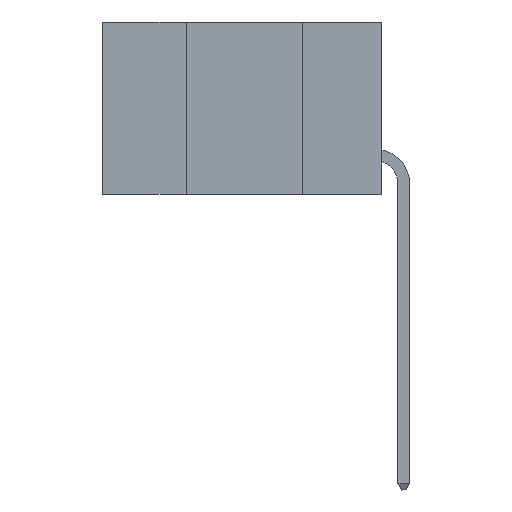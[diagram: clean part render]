
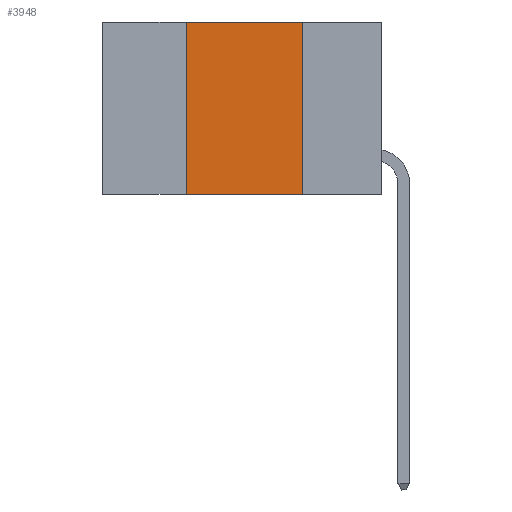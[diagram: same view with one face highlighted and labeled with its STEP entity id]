
A CAD part, left-side view. The second image highlights one B-rep face of the part: STEP entity #3948.
In plain terms, the highlighted planar face has unit normal (-1, 0, 0).
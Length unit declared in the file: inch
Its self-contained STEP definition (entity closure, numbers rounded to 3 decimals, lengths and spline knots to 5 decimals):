
#1010 = LINE ( 'NONE', #6924, #2339 ) ;
#1045 = DIRECTION ( 'NONE',  ( 1., 0., 0. ) ) ;
#1065 = ORIENTED_EDGE ( 'NONE', *, *, #8883, .F. ) ;
#1316 = CARTESIAN_POINT ( 'NONE',  ( 0., 0.17, 0. ) ) ;
#1758 = VECTOR ( 'NONE', #2077, 39.37008 ) ;
#1809 = PLANE ( 'NONE',  #6838 ) ;
#2077 = DIRECTION ( 'NONE',  ( 0., 0., -1. ) ) ;
#2259 = ORIENTED_EDGE ( 'NONE', *, *, #10439, .F. ) ;
#2339 = VECTOR ( 'NONE', #3512, 39.37008 ) ;
#2838 = CARTESIAN_POINT ( 'NONE',  ( 0., 0.17, -0.37 ) ) ;
#2839 = FACE_OUTER_BOUND ( 'NONE', #4498, .T. ) ;
#3044 = DIRECTION ( 'NONE',  ( 0., 0., 1. ) ) ;
#3199 = VECTOR ( 'NONE', #3044, 39.37008 ) ;
#3502 = DIRECTION ( 'NONE',  ( 0., 0., -1. ) ) ;
#3512 = DIRECTION ( 'NONE',  ( 0., -1., 0. ) ) ;
#3948 = ADVANCED_FACE ( 'NONE', ( #2839 ), #1809, .F. ) ;
#4498 = EDGE_LOOP ( 'NONE', ( #2259, #1065, #7456, #8325 ) ) ;
#4534 = VECTOR ( 'NONE', #10277, 39.37008 ) ;
#4605 = CARTESIAN_POINT ( 'NONE',  ( 0., 0.17, 0. ) ) ;
#4914 = EDGE_CURVE ( 'NONE', #10272, #5279, #5038, .T. ) ;
#5038 = LINE ( 'NONE', #10020, #4534 ) ;
#5279 = VERTEX_POINT ( 'NONE', #2838 ) ;
#5331 = CARTESIAN_POINT ( 'NONE',  ( 0., 0.42, 0. ) ) ;
#5947 = LINE ( 'NONE', #4605, #1758 ) ;
#6838 = AXIS2_PLACEMENT_3D ( 'NONE', #7599, #1045, #3502 ) ;
#6924 = CARTESIAN_POINT ( 'NONE',  ( 0., 0.6, 0. ) ) ;
#7456 = ORIENTED_EDGE ( 'NONE', *, *, #10737, .F. ) ;
#7599 = CARTESIAN_POINT ( 'NONE',  ( 0., 0.6, 0. ) ) ;
#8325 = ORIENTED_EDGE ( 'NONE', *, *, #4914, .T. ) ;
#8883 = EDGE_CURVE ( 'NONE', #9912, #9751, #1010, .T. ) ;
#9596 = LINE ( 'NONE', #9688, #3199 ) ;
#9688 = CARTESIAN_POINT ( 'NONE',  ( 0., 0.42, 0. ) ) ;
#9751 = VERTEX_POINT ( 'NONE', #1316 ) ;
#9912 = VERTEX_POINT ( 'NONE', #5331 ) ;
#10020 = CARTESIAN_POINT ( 'NONE',  ( 0., 0.6, -0.37 ) ) ;
#10150 = CARTESIAN_POINT ( 'NONE',  ( 0., 0.42, -0.37 ) ) ;
#10272 = VERTEX_POINT ( 'NONE', #10150 ) ;
#10277 = DIRECTION ( 'NONE',  ( 0., -1., 0. ) ) ;
#10439 = EDGE_CURVE ( 'NONE', #9751, #5279, #5947, .T. ) ;
#10737 = EDGE_CURVE ( 'NONE', #10272, #9912, #9596, .T. ) ;
